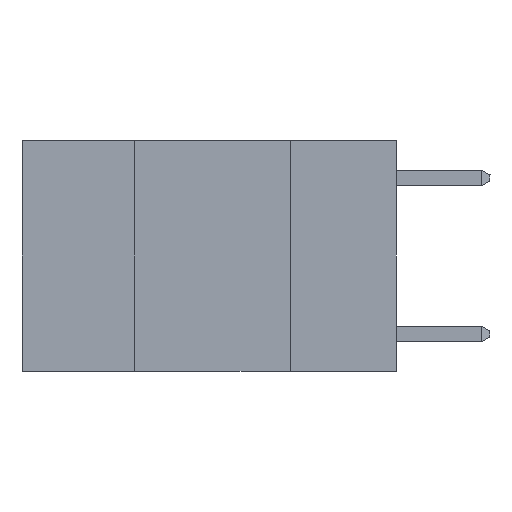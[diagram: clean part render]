
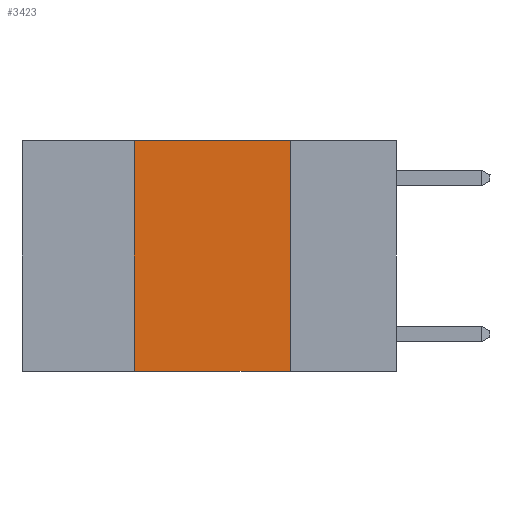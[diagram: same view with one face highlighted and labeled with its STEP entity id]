
A CAD part, left-side view. The second image highlights one B-rep face of the part: STEP entity #3423.
In plain terms, the highlighted planar face has unit normal (-1, 0, 0).
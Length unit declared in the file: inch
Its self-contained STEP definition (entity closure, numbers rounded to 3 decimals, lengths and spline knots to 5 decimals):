
#628 = EDGE_CURVE ( 'NONE', #10167, #8428, #2011, .T. ) ;
#934 = CARTESIAN_POINT ( 'NONE',  ( 0., 0.17, -0.37 ) ) ;
#1442 = VECTOR ( 'NONE', #6052, 39.37008 ) ;
#1823 = ORIENTED_EDGE ( 'NONE', *, *, #7692, .F. ) ;
#2011 = LINE ( 'NONE', #8650, #11367 ) ;
#2677 = CARTESIAN_POINT ( 'NONE',  ( 0., 0.6, 0. ) ) ;
#3383 = ORIENTED_EDGE ( 'NONE', *, *, #5227, .F. ) ;
#3404 = ORIENTED_EDGE ( 'NONE', *, *, #628, .F. ) ;
#3423 = ADVANCED_FACE ( 'NONE', ( #7418 ), #6437, .F. ) ;
#3634 = CARTESIAN_POINT ( 'NONE',  ( 0., 0.6, -0.37 ) ) ;
#3642 = DIRECTION ( 'NONE',  ( 0., 0., -1. ) ) ;
#4020 = DIRECTION ( 'NONE',  ( 0., 0., 1. ) ) ;
#4849 = CARTESIAN_POINT ( 'NONE',  ( 0., 0.17, 0. ) ) ;
#5227 = EDGE_CURVE ( 'NONE', #8428, #5497, #8246, .T. ) ;
#5230 = VECTOR ( 'NONE', #9187, 39.37008 ) ;
#5464 = VERTEX_POINT ( 'NONE', #934 ) ;
#5492 = VECTOR ( 'NONE', #10961, 39.37008 ) ;
#5497 = VERTEX_POINT ( 'NONE', #4849 ) ;
#5524 = LINE ( 'NONE', #3634, #5230 ) ;
#6052 = DIRECTION ( 'NONE',  ( 0., 0., -1. ) ) ;
#6247 = LINE ( 'NONE', #9791, #1442 ) ;
#6437 = PLANE ( 'NONE',  #8198 ) ;
#6656 = EDGE_CURVE ( 'NONE', #10167, #5464, #5524, .T. ) ;
#6764 = CARTESIAN_POINT ( 'NONE',  ( 0., 0.42, -0.37 ) ) ;
#7418 = FACE_OUTER_BOUND ( 'NONE', #11747, .T. ) ;
#7692 = EDGE_CURVE ( 'NONE', #5497, #5464, #6247, .T. ) ;
#8198 = AXIS2_PLACEMENT_3D ( 'NONE', #2677, #9237, #3642 ) ;
#8246 = LINE ( 'NONE', #11820, #5492 ) ;
#8428 = VERTEX_POINT ( 'NONE', #10095 ) ;
#8650 = CARTESIAN_POINT ( 'NONE',  ( 0., 0.42, 0. ) ) ;
#9153 = ORIENTED_EDGE ( 'NONE', *, *, #6656, .T. ) ;
#9187 = DIRECTION ( 'NONE',  ( 0., -1., 0. ) ) ;
#9237 = DIRECTION ( 'NONE',  ( 1., 0., 0. ) ) ;
#9791 = CARTESIAN_POINT ( 'NONE',  ( 0., 0.17, 0. ) ) ;
#10095 = CARTESIAN_POINT ( 'NONE',  ( 0., 0.42, 0. ) ) ;
#10167 = VERTEX_POINT ( 'NONE', #6764 ) ;
#10961 = DIRECTION ( 'NONE',  ( 0., -1., 0. ) ) ;
#11367 = VECTOR ( 'NONE', #4020, 39.37008 ) ;
#11747 = EDGE_LOOP ( 'NONE', ( #1823, #3383, #3404, #9153 ) ) ;
#11820 = CARTESIAN_POINT ( 'NONE',  ( 0., 0.6, 0. ) ) ;
